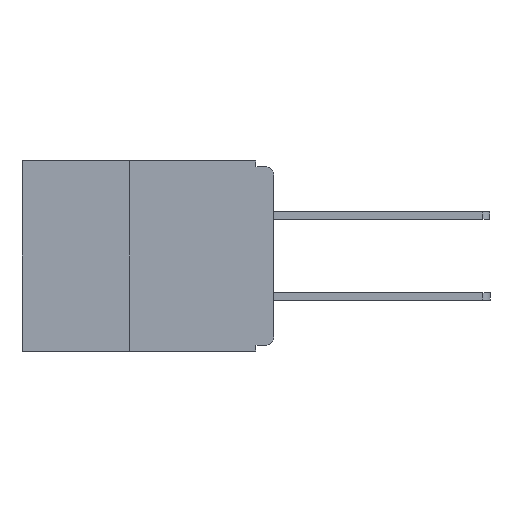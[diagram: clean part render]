
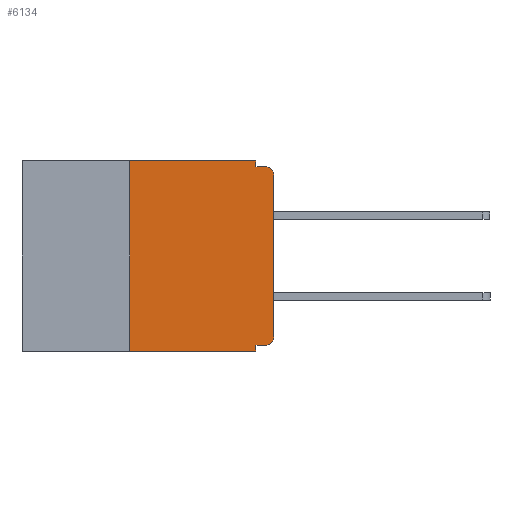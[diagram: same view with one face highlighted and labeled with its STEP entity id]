
A CAD part, left-side view. The second image highlights one B-rep face of the part: STEP entity #6134.
In plain terms, the highlighted planar face has unit normal (-1, 0, 0).
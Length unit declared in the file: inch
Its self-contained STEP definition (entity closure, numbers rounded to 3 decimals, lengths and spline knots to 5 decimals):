
#134 = CARTESIAN_POINT ( 'NONE',  ( 0., 0.031, -0.33 ) ) ;
#418 = DIRECTION ( 'NONE',  ( 0., 0., -1. ) ) ;
#461 = DIRECTION ( 'NONE',  ( -1., 0., 0. ) ) ;
#479 = CARTESIAN_POINT ( 'NONE',  ( 0., 0.015, -0.025 ) ) ;
#551 = CARTESIAN_POINT ( 'NONE',  ( 0., 0., -0.32 ) ) ;
#1201 = EDGE_CURVE ( 'NONE', #7594, #9703, #2287, .T. ) ;
#1419 = DIRECTION ( 'NONE',  ( 0., 0., -1. ) ) ;
#1802 = ORIENTED_EDGE ( 'NONE', *, *, #10207, .F. ) ;
#1925 = ORIENTED_EDGE ( 'NONE', *, *, #15659, .F. ) ;
#1991 = VERTEX_POINT ( 'NONE', #13664 ) ;
#2224 = LINE ( 'NONE', #134, #9643 ) ;
#2287 = CIRCLE ( 'NONE', #17461, 0.015 ) ;
#2353 = VERTEX_POINT ( 'NONE', #10849 ) ;
#3159 = DIRECTION ( 'NONE',  ( 0., 0., -1. ) ) ;
#3384 = DIRECTION ( 'NONE',  ( -1., 0., 0. ) ) ;
#3470 = EDGE_CURVE ( 'NONE', #5697, #2353, #2224, .T. ) ;
#3764 = CARTESIAN_POINT ( 'NONE',  ( 0., 0.015, -0.305 ) ) ;
#3838 = CARTESIAN_POINT ( 'NONE',  ( 0., 0., -0.305 ) ) ;
#3962 = VECTOR ( 'NONE', #10422, 39.37008 ) ;
#4025 = VERTEX_POINT ( 'NONE', #17036 ) ;
#4394 = VERTEX_POINT ( 'NONE', #9304 ) ;
#4498 = EDGE_CURVE ( 'NONE', #4394, #2353, #18452, .T. ) ;
#5019 = EDGE_CURVE ( 'NONE', #9703, #15337, #6140, .T. ) ;
#5491 = LINE ( 'NONE', #13260, #9305 ) ;
#5506 = EDGE_CURVE ( 'NONE', #4394, #12455, #13678, .T. ) ;
#5553 = ORIENTED_EDGE ( 'NONE', *, *, #14861, .F. ) ;
#5697 = VERTEX_POINT ( 'NONE', #15191 ) ;
#6121 = VECTOR ( 'NONE', #16776, 39.37008 ) ;
#6134 = ADVANCED_FACE ( 'NONE', ( #17191 ), #11570, .F. ) ;
#6140 = LINE ( 'NONE', #6158, #16791 ) ;
#6158 = CARTESIAN_POINT ( 'NONE',  ( 0., 0., 0. ) ) ;
#6165 = DIRECTION ( 'NONE',  ( 0., -1., 0. ) ) ;
#6363 = DIRECTION ( 'NONE',  ( 0., 0., 1. ) ) ;
#6383 = ORIENTED_EDGE ( 'NONE', *, *, #4498, .T. ) ;
#6412 = ORIENTED_EDGE ( 'NONE', *, *, #3470, .F. ) ;
#7325 = EDGE_CURVE ( 'NONE', #15337, #1991, #13419, .T. ) ;
#7372 = ORIENTED_EDGE ( 'NONE', *, *, #5019, .T. ) ;
#7431 = EDGE_CURVE ( 'NONE', #14588, #4025, #8309, .T. ) ;
#7512 = VECTOR ( 'NONE', #17735, 39.37008 ) ;
#7594 = VERTEX_POINT ( 'NONE', #17031 ) ;
#8003 = AXIS2_PLACEMENT_3D ( 'NONE', #11463, #11459, #11438 ) ;
#8309 = LINE ( 'NONE', #16610, #3962 ) ;
#9304 = CARTESIAN_POINT ( 'NONE',  ( 0., 0.25, -0.33 ) ) ;
#9305 = VECTOR ( 'NONE', #6165, 39.37008 ) ;
#9338 = LINE ( 'NONE', #14195, #13114 ) ;
#9439 = AXIS2_PLACEMENT_3D ( 'NONE', #479, #461, #418 ) ;
#9643 = VECTOR ( 'NONE', #1419, 39.37008 ) ;
#9674 = CARTESIAN_POINT ( 'NONE',  ( 0., 0., -0.025 ) ) ;
#9703 = VERTEX_POINT ( 'NONE', #3838 ) ;
#10207 = EDGE_CURVE ( 'NONE', #7594, #5697, #11365, .T. ) ;
#10422 = DIRECTION ( 'NONE',  ( 0., 0., -1. ) ) ;
#10849 = CARTESIAN_POINT ( 'NONE',  ( 0., 0.031, -0.33 ) ) ;
#10993 = DIRECTION ( 'NONE',  ( 0., 1., 0. ) ) ;
#11365 = LINE ( 'NONE', #551, #18469 ) ;
#11433 = DIRECTION ( 'NONE',  ( 0., -1., 0. ) ) ;
#11438 = DIRECTION ( 'NONE',  ( 0., 0., -1. ) ) ;
#11459 = DIRECTION ( 'NONE',  ( 1., 0., 0. ) ) ;
#11463 = CARTESIAN_POINT ( 'NONE',  ( 0., 0.437, 0. ) ) ;
#11500 = ORIENTED_EDGE ( 'NONE', *, *, #1201, .T. ) ;
#11570 = PLANE ( 'NONE',  #8003 ) ;
#11984 = EDGE_LOOP ( 'NONE', ( #7372, #14980, #5553, #16475, #1925, #17906, #6383, #6412, #1802, #11500 ) ) ;
#12455 = VERTEX_POINT ( 'NONE', #13195 ) ;
#13114 = VECTOR ( 'NONE', #11433, 39.37008 ) ;
#13195 = CARTESIAN_POINT ( 'NONE',  ( 0., 0.25, 0. ) ) ;
#13260 = CARTESIAN_POINT ( 'NONE',  ( 0., 0.437, 0. ) ) ;
#13419 = CIRCLE ( 'NONE', #9439, 0.015 ) ;
#13548 = CARTESIAN_POINT ( 'NONE',  ( 0., 0.031, 0. ) ) ;
#13664 = CARTESIAN_POINT ( 'NONE',  ( 0., 0.015, -0.01 ) ) ;
#13678 = LINE ( 'NONE', #16917, #6121 ) ;
#14195 = CARTESIAN_POINT ( 'NONE',  ( 0., 0., -0.01 ) ) ;
#14588 = VERTEX_POINT ( 'NONE', #13548 ) ;
#14861 = EDGE_CURVE ( 'NONE', #4025, #1991, #9338, .T. ) ;
#14980 = ORIENTED_EDGE ( 'NONE', *, *, #7325, .T. ) ;
#15191 = CARTESIAN_POINT ( 'NONE',  ( 0., 0.031, -0.32 ) ) ;
#15337 = VERTEX_POINT ( 'NONE', #9674 ) ;
#15659 = EDGE_CURVE ( 'NONE', #12455, #14588, #5491, .T. ) ;
#16475 = ORIENTED_EDGE ( 'NONE', *, *, #7431, .F. ) ;
#16610 = CARTESIAN_POINT ( 'NONE',  ( 0., 0.031, 0. ) ) ;
#16776 = DIRECTION ( 'NONE',  ( 0., 0., 1. ) ) ;
#16791 = VECTOR ( 'NONE', #6363, 39.37008 ) ;
#16917 = CARTESIAN_POINT ( 'NONE',  ( 0., 0.25, -0.33 ) ) ;
#17031 = CARTESIAN_POINT ( 'NONE',  ( 0., 0.015, -0.32 ) ) ;
#17036 = CARTESIAN_POINT ( 'NONE',  ( 0., 0.031, -0.01 ) ) ;
#17191 = FACE_OUTER_BOUND ( 'NONE', #11984, .T. ) ;
#17273 = CARTESIAN_POINT ( 'NONE',  ( 0., 0.437, -0.33 ) ) ;
#17461 = AXIS2_PLACEMENT_3D ( 'NONE', #3764, #3384, #3159 ) ;
#17735 = DIRECTION ( 'NONE',  ( 0., -1., 0. ) ) ;
#17906 = ORIENTED_EDGE ( 'NONE', *, *, #5506, .F. ) ;
#18452 = LINE ( 'NONE', #17273, #7512 ) ;
#18469 = VECTOR ( 'NONE', #10993, 39.37008 ) ;
